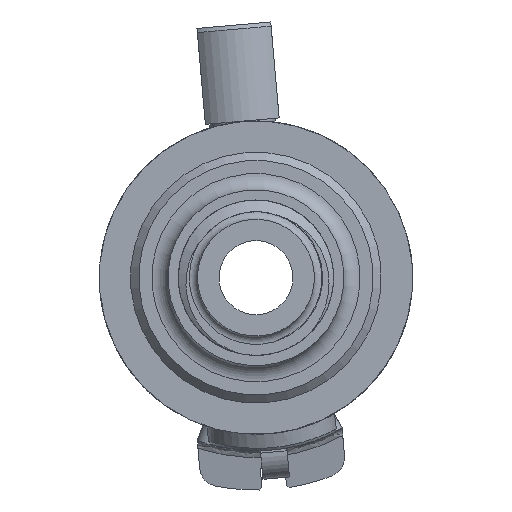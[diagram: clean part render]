
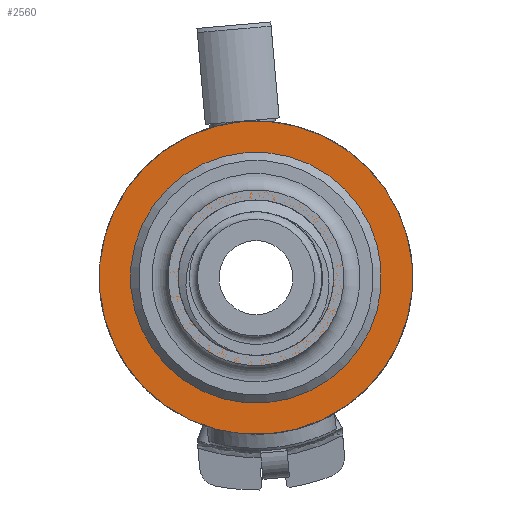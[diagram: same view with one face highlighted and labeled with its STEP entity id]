
A CAD part, left-side view. The second image highlights one B-rep face of the part: STEP entity #2560.
In plain terms, the highlighted planar face has unit normal (-1, 0, 0).
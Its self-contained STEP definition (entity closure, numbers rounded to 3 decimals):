
#76=CIRCLE('',#2732,19.05);
#91=CIRCLE('',#2777,4.5);
#153=FACE_BOUND('',#540,.T.);
#256=PLANE('',#2779);
#379=FACE_OUTER_BOUND('',#539,.T.);
#539=EDGE_LOOP('',(#2263));
#540=EDGE_LOOP('',(#2264));
#1181=VERTEX_POINT('',#12790);
#1230=VERTEX_POINT('',#13224);
#1509=EDGE_CURVE('',#1181,#1181,#76,.T.);
#1582=EDGE_CURVE('',#1230,#1230,#91,.T.);
#2263=ORIENTED_EDGE('',*,*,#1509,.T.);
#2264=ORIENTED_EDGE('',*,*,#1582,.T.);
#2560=ADVANCED_FACE('',(#379,#153),#256,.T.);
#2732=AXIS2_PLACEMENT_3D('',#12791,#3147,#3148);
#2777=AXIS2_PLACEMENT_3D('',#13225,#3273,#3274);
#2779=AXIS2_PLACEMENT_3D('',#13229,#3279,#3280);
#3147=DIRECTION('center_axis',(-1.,0.,0.));
#3148=DIRECTION('ref_axis',(0.,0.966,-0.259));
#3273=DIRECTION('center_axis',(1.,0.,0.));
#3274=DIRECTION('ref_axis',(0.,-0.996,0.087));
#3279=DIRECTION('center_axis',(-1.,0.,0.));
#3280=DIRECTION('ref_axis',(0.,-0.996,0.087));
#12790=CARTESIAN_POINT('',(-84.5,-18.401,-96.069));
#12791=CARTESIAN_POINT('Origin',(-84.5,0.,-101.));
#13224=CARTESIAN_POINT('',(-84.5,4.483,-101.392));
#13225=CARTESIAN_POINT('Origin',(-84.5,0.,-101.));
#13229=CARTESIAN_POINT('Origin',(-84.5,0.009,-100.9));
